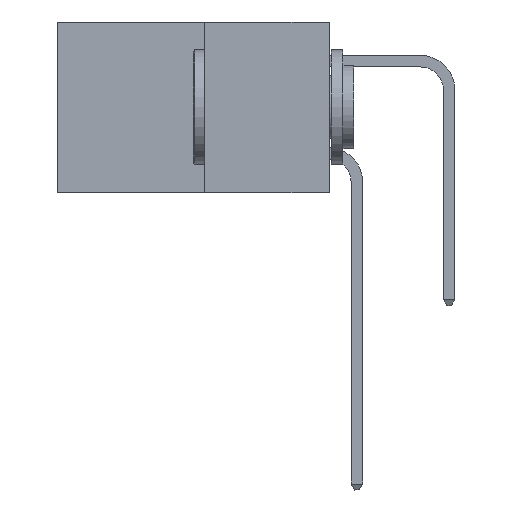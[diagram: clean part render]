
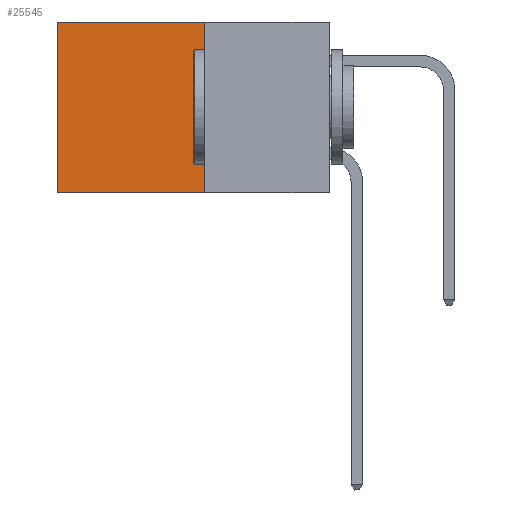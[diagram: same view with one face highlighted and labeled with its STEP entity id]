
A CAD part, left-side view. The second image highlights one B-rep face of the part: STEP entity #25545.
In plain terms, the highlighted planar face has unit normal (-1, 0, 0).
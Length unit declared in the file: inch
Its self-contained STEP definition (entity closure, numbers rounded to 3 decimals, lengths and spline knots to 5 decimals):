
#117 = ORIENTED_EDGE ( 'NONE', *, *, #14448, .F. ) ;
#1201 = AXIS2_PLACEMENT_3D ( 'NONE', #7822, #10440, #28475 ) ;
#1848 = VECTOR ( 'NONE', #10034, 39.37008 ) ;
#3034 = ORIENTED_EDGE ( 'NONE', *, *, #32064, .T. ) ;
#4123 = FACE_OUTER_BOUND ( 'NONE', #6303, .T. ) ;
#4435 = CARTESIAN_POINT ( 'NONE',  ( 0.277, 0.27, -0.37 ) ) ;
#5127 = VECTOR ( 'NONE', #24536, 39.37008 ) ;
#5187 = PLANE ( 'NONE',  #1201 ) ;
#5593 = VERTEX_POINT ( 'NONE', #29118 ) ;
#6303 = EDGE_LOOP ( 'NONE', ( #30630, #117, #14311, #3034 ) ) ;
#7419 = CARTESIAN_POINT ( 'NONE',  ( 0.277, 0.59, -0.37 ) ) ;
#7822 = CARTESIAN_POINT ( 'NONE',  ( 0.277, 0.27, -0.37 ) ) ;
#8526 = CARTESIAN_POINT ( 'NONE',  ( 0.277, 0.27, -0.37 ) ) ;
#8586 = VERTEX_POINT ( 'NONE', #8526 ) ;
#10034 = DIRECTION ( 'NONE',  ( 0., 0., -1. ) ) ;
#10440 = DIRECTION ( 'NONE',  ( 1., 0., 0. ) ) ;
#14311 = ORIENTED_EDGE ( 'NONE', *, *, #14973, .F. ) ;
#14448 = EDGE_CURVE ( 'NONE', #8586, #27667, #28227, .T. ) ;
#14973 = EDGE_CURVE ( 'NONE', #25971, #8586, #25775, .T. ) ;
#15358 = VECTOR ( 'NONE', #22549, 39.37008 ) ;
#15541 = CARTESIAN_POINT ( 'NONE',  ( 0.277, 0.59, -0.37 ) ) ;
#16815 = DIRECTION ( 'NONE',  ( 0., 1., 0. ) ) ;
#17480 = VECTOR ( 'NONE', #16815, 39.37008 ) ;
#21981 = CARTESIAN_POINT ( 'NONE',  ( 0.277, 0.27, -0.37 ) ) ;
#22538 = LINE ( 'NONE', #7419, #1848 ) ;
#22549 = DIRECTION ( 'NONE',  ( 0., 1., 0. ) ) ;
#24308 = LINE ( 'NONE', #24443, #17480 ) ;
#24443 = CARTESIAN_POINT ( 'NONE',  ( 0.277, 0.27, 0. ) ) ;
#24536 = DIRECTION ( 'NONE',  ( 0., 0., -1. ) ) ;
#25545 = ADVANCED_FACE ( 'NONE', ( #4123 ), #5187, .F. ) ;
#25775 = LINE ( 'NONE', #21981, #5127 ) ;
#25971 = VERTEX_POINT ( 'NONE', #27329 ) ;
#27329 = CARTESIAN_POINT ( 'NONE',  ( 0.277, 0.27, 0. ) ) ;
#27667 = VERTEX_POINT ( 'NONE', #15541 ) ;
#28227 = LINE ( 'NONE', #4435, #15358 ) ;
#28475 = DIRECTION ( 'NONE',  ( 0., 0., -1. ) ) ;
#28811 = EDGE_CURVE ( 'NONE', #5593, #27667, #22538, .T. ) ;
#29118 = CARTESIAN_POINT ( 'NONE',  ( 0.277, 0.59, 0. ) ) ;
#30630 = ORIENTED_EDGE ( 'NONE', *, *, #28811, .T. ) ;
#32064 = EDGE_CURVE ( 'NONE', #25971, #5593, #24308, .T. ) ;
